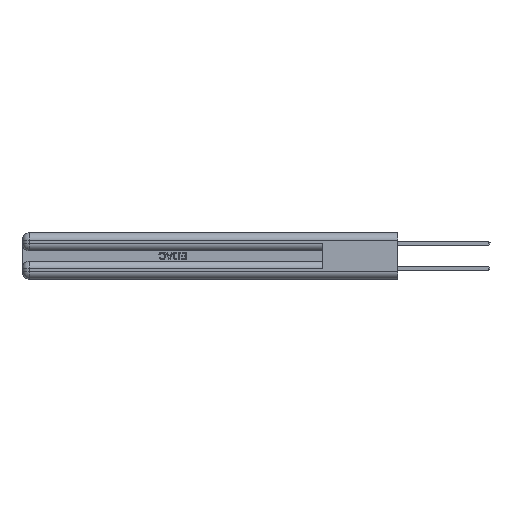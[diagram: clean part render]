
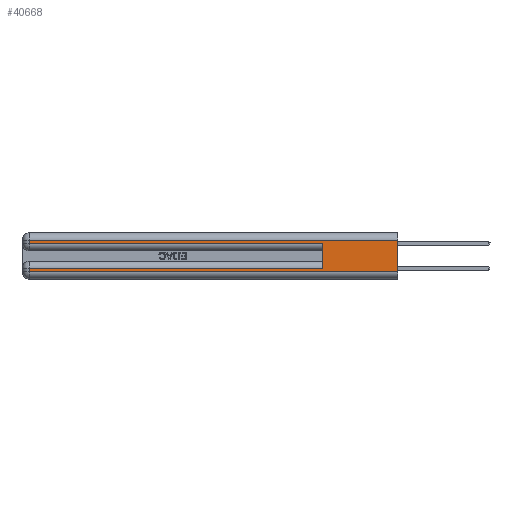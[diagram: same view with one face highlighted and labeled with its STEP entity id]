
A CAD part, left-side view. The second image highlights one B-rep face of the part: STEP entity #40668.
In plain terms, the highlighted planar face has unit normal (-1, 0, 0).
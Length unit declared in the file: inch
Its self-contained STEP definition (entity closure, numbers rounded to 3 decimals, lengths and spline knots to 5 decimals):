
#194 = VECTOR ( 'NONE', #24835, 39.37008 ) ;
#681 = VERTEX_POINT ( 'NONE', #24391 ) ;
#762 = EDGE_CURVE ( 'NONE', #890, #43469, #23914, .T. ) ;
#890 = VERTEX_POINT ( 'NONE', #13079 ) ;
#2099 = ORIENTED_EDGE ( 'NONE', *, *, #762, .F. ) ;
#2885 = DIRECTION ( 'NONE',  ( 0., -1., 0. ) ) ;
#4034 = LINE ( 'NONE', #8067, #194 ) ;
#4758 = CARTESIAN_POINT ( 'NONE',  ( 0., 0.6, 0.285 ) ) ;
#5827 = VECTOR ( 'NONE', #7655, 39.37008 ) ;
#7468 = CARTESIAN_POINT ( 'NONE',  ( 0., 0., 0.06 ) ) ;
#7540 = AXIS2_PLACEMENT_3D ( 'NONE', #30235, #14180, #21622 ) ;
#7655 = DIRECTION ( 'NONE',  ( 0., 0., 1. ) ) ;
#8067 = CARTESIAN_POINT ( 'NONE',  ( 0., 2.94, 0.37 ) ) ;
#9761 = PLANE ( 'NONE',  #7540 ) ;
#10724 = CARTESIAN_POINT ( 'NONE',  ( 0., 2.94, 0.06 ) ) ;
#10780 = LINE ( 'NONE', #23441, #39176 ) ;
#12416 = EDGE_CURVE ( 'NONE', #681, #23222, #4034, .T. ) ;
#13079 = CARTESIAN_POINT ( 'NONE',  ( 0., 0., 0.31 ) ) ;
#13508 = FACE_OUTER_BOUND ( 'NONE', #14002, .T. ) ;
#13757 = VECTOR ( 'NONE', #48003, 39.37008 ) ;
#14002 = EDGE_LOOP ( 'NONE', ( #2099, #20817, #36749, #20581, #42346, #33686, #38718, #49191 ) ) ;
#14180 = DIRECTION ( 'NONE',  ( 1., 0., 0. ) ) ;
#17420 = VECTOR ( 'NONE', #2885, 39.37008 ) ;
#17713 = VECTOR ( 'NONE', #43465, 39.37008 ) ;
#18252 = VERTEX_POINT ( 'NONE', #10724 ) ;
#19058 = LINE ( 'NONE', #32797, #32940 ) ;
#20011 = EDGE_CURVE ( 'NONE', #50222, #18252, #20477, .T. ) ;
#20477 = LINE ( 'NONE', #33206, #28662 ) ;
#20581 = ORIENTED_EDGE ( 'NONE', *, *, #31040, .T. ) ;
#20817 = ORIENTED_EDGE ( 'NONE', *, *, #34769, .T. ) ;
#21622 = DIRECTION ( 'NONE',  ( 0., 0., -1. ) ) ;
#23222 = VERTEX_POINT ( 'NONE', #23597 ) ;
#23441 = CARTESIAN_POINT ( 'NONE',  ( 0., 0., 0.085 ) ) ;
#23597 = CARTESIAN_POINT ( 'NONE',  ( 0., 2.94, 0.285 ) ) ;
#23914 = LINE ( 'NONE', #48350, #13757 ) ;
#24391 = CARTESIAN_POINT ( 'NONE',  ( 0., 2.94, 0.31 ) ) ;
#24835 = DIRECTION ( 'NONE',  ( 0., 0., -1. ) ) ;
#24856 = DIRECTION ( 'NONE',  ( 0., 1., 0. ) ) ;
#26897 = CARTESIAN_POINT ( 'NONE',  ( 0., 0., 0.285 ) ) ;
#27811 = EDGE_CURVE ( 'NONE', #51970, #50222, #10780, .T. ) ;
#28143 = CARTESIAN_POINT ( 'NONE',  ( 0., 0.6, 0.145 ) ) ;
#28498 = EDGE_CURVE ( 'NONE', #18252, #43469, #50462, .T. ) ;
#28662 = VECTOR ( 'NONE', #49912, 39.37008 ) ;
#30235 = CARTESIAN_POINT ( 'NONE',  ( 0., 0., 0.37 ) ) ;
#31040 = EDGE_CURVE ( 'NONE', #23222, #50201, #37615, .T. ) ;
#32797 = CARTESIAN_POINT ( 'NONE',  ( 0., 0., 0.31 ) ) ;
#32940 = VECTOR ( 'NONE', #24856, 39.37008 ) ;
#32976 = LINE ( 'NONE', #28143, #5827 ) ;
#33206 = CARTESIAN_POINT ( 'NONE',  ( 0., 2.94, 0.37 ) ) ;
#33686 = ORIENTED_EDGE ( 'NONE', *, *, #27811, .T. ) ;
#34769 = EDGE_CURVE ( 'NONE', #890, #681, #19058, .T. ) ;
#36749 = ORIENTED_EDGE ( 'NONE', *, *, #12416, .T. ) ;
#37615 = LINE ( 'NONE', #26897, #17420 ) ;
#38718 = ORIENTED_EDGE ( 'NONE', *, *, #20011, .T. ) ;
#38805 = CARTESIAN_POINT ( 'NONE',  ( 0., 0.6, 0.085 ) ) ;
#39176 = VECTOR ( 'NONE', #51654, 39.37008 ) ;
#40668 = ADVANCED_FACE ( 'NONE', ( #13508 ), #9761, .F. ) ;
#41803 = EDGE_CURVE ( 'NONE', #51970, #50201, #32976, .T. ) ;
#42346 = ORIENTED_EDGE ( 'NONE', *, *, #41803, .F. ) ;
#43465 = DIRECTION ( 'NONE',  ( 0., -1., 0. ) ) ;
#43469 = VERTEX_POINT ( 'NONE', #47362 ) ;
#47362 = CARTESIAN_POINT ( 'NONE',  ( 0., 0., 0.06 ) ) ;
#48003 = DIRECTION ( 'NONE',  ( 0., 0., -1. ) ) ;
#48350 = CARTESIAN_POINT ( 'NONE',  ( 0., 0., 0.37 ) ) ;
#48672 = CARTESIAN_POINT ( 'NONE',  ( 0., 2.94, 0.085 ) ) ;
#49191 = ORIENTED_EDGE ( 'NONE', *, *, #28498, .T. ) ;
#49912 = DIRECTION ( 'NONE',  ( 0., 0., -1. ) ) ;
#50201 = VERTEX_POINT ( 'NONE', #4758 ) ;
#50222 = VERTEX_POINT ( 'NONE', #48672 ) ;
#50462 = LINE ( 'NONE', #7468, #17713 ) ;
#51654 = DIRECTION ( 'NONE',  ( 0., 1., 0. ) ) ;
#51970 = VERTEX_POINT ( 'NONE', #38805 ) ;
